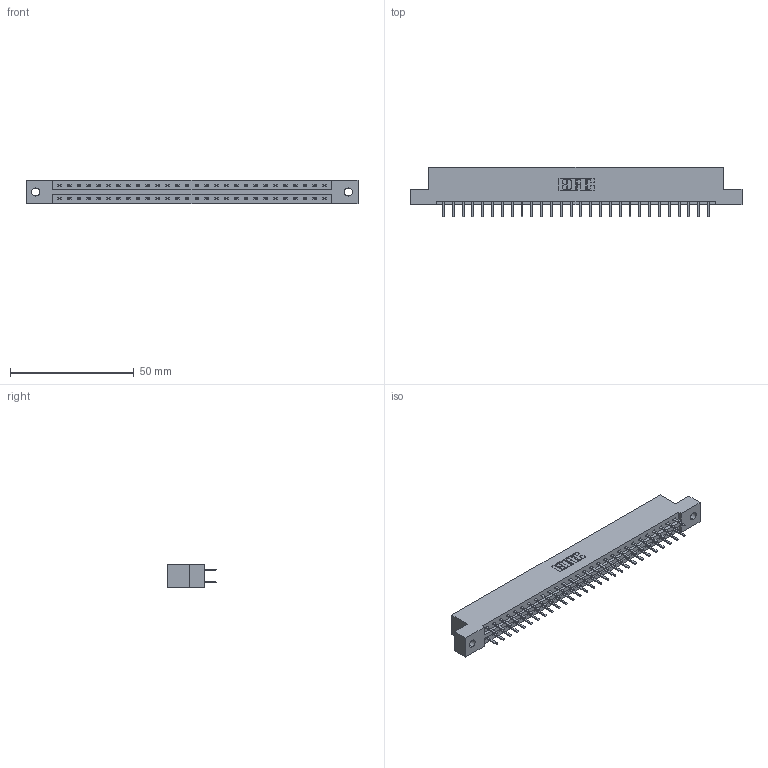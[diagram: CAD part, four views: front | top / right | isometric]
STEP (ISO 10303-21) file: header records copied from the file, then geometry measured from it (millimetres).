
FILE_DESCRIPTION (( 'STEP AP203' ), '1' );
FILE_NAME ('337-056-520-202.STEP', '2018-08-10T02:12:15', ( '' ), ( '' ), 'SwSTEP 2.0', 'SolidWorks 2016', '' );
FILE_SCHEMA (( 'CONFIG_CONTROL_DESIGN' ));
Length unit declared in the file: inch
Products named in the file (3): 337 Part_Flush Mounting Lugs - 0.128 Dia; 345-292-001_345-293-120; 337-056-520-202
Assembly tree (57 placements, depth 2):
  337-056-520-202
    337 Part_Flush Mounting Lugs - 0.128 Dia
    345-292-001_345-293-120  x56
Bounding box: 133.96 x 20.02 x 9.4 mm (x, y, z)
Volume: 13870.1 mm3; surface area: 15201.2 mm2
Topology: 57 solids, 57 shells, 3362 faces, 9775 edges, 6366 vertices
Faces by surface type: plane 2310, cylinder 1052
Entity records: 23637 total; most frequent: CARTESIAN_POINT 4006, ORIENTED_EDGE 3930, DIRECTION 3421, EDGE_CURVE 1965, VECTOR 1833, LINE 1833, VERTEX_POINT 1306, AXIS2_PLACEMENT_3D 794
